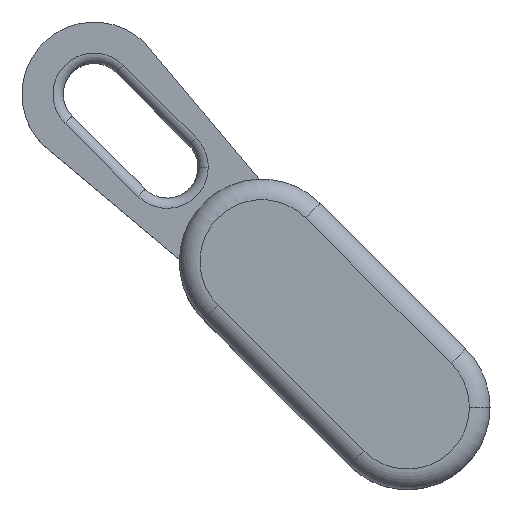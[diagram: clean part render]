
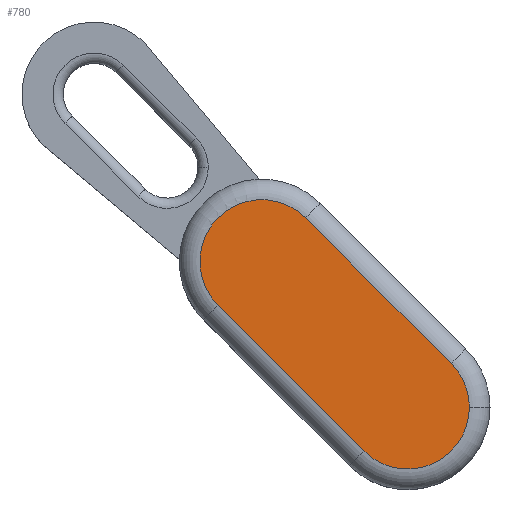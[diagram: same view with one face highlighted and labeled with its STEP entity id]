
A CAD part, top view. The second image highlights one B-rep face of the part: STEP entity #780.
In plain terms, the highlighted planar face has unit normal (0, 0, 1).
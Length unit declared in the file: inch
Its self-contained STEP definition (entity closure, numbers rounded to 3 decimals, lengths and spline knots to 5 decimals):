
#4 = LINE ( 'NONE', #645, #909 ) ;
#46 = FACE_OUTER_BOUND ( 'NONE', #1420, .T. ) ;
#127 = DIRECTION ( 'NONE',  ( 0.707, -0.707, 0. ) ) ;
#155 = VERTEX_POINT ( 'NONE', #1079 ) ;
#251 = DIRECTION ( 'NONE',  ( 0., 0., 1. ) ) ;
#254 = CIRCLE ( 'NONE', #668, 0.11811 ) ;
#264 = EDGE_CURVE ( 'NONE', #755, #1204, #975, .T. ) ;
#313 = DIRECTION ( 'NONE',  ( 0., 0., 1. ) ) ;
#320 = CARTESIAN_POINT ( 'NONE',  ( 0.55657, -0.50477, 0.61024 ) ) ;
#396 = CARTESIAN_POINT ( 'NONE',  ( 0.16007, -0.22638, 0.61024 ) ) ;
#404 = DIRECTION ( 'NONE',  ( 0., 0., 1. ) ) ;
#526 = DIRECTION ( 'NONE',  ( 1., 0., 0. ) ) ;
#633 = LINE ( 'NONE', #1086, #1436 ) ;
#645 = CARTESIAN_POINT ( 'NONE',  ( 0.05036, 0.05036, 0.61024 ) ) ;
#668 = AXIS2_PLACEMENT_3D ( 'NONE', #1092, #404, #1200 ) ;
#702 = AXIS2_PLACEMENT_3D ( 'NONE', #396, #1196, #526 ) ;
#755 = VERTEX_POINT ( 'NONE', #1172 ) ;
#763 = DIRECTION ( 'NONE',  ( -0.707, 0.707, 0. ) ) ;
#780 = ADVANCED_FACE ( 'NONE', ( #46 ), #971, .T. ) ;
#805 = EDGE_CURVE ( 'NONE', #1356, #155, #4, .T. ) ;
#812 = EDGE_CURVE ( 'NONE', #155, #1235, #1184, .T. ) ;
#817 = EDGE_CURVE ( 'NONE', #1235, #755, #633, .T. ) ;
#835 = EDGE_CURVE ( 'NONE', #1204, #1356, #254, .T. ) ;
#867 = CARTESIAN_POINT ( 'NONE',  ( 0., 0., 0.61024 ) ) ;
#909 = VECTOR ( 'NONE', #763, 39.37008 ) ;
#920 = ORIENTED_EDGE ( 'NONE', *, *, #264, .T. ) ;
#952 = ORIENTED_EDGE ( 'NONE', *, *, #805, .T. ) ;
#964 = AXIS2_PLACEMENT_3D ( 'NONE', #867, #251, #1077 ) ;
#971 = PLANE ( 'NONE',  #964 ) ;
#975 = CIRCLE ( 'NONE', #1213, 0.11811 ) ;
#1021 = CARTESIAN_POINT ( 'NONE',  ( 0.43846, -0.50477, 0.61024 ) ) ;
#1033 = CARTESIAN_POINT ( 'NONE',  ( 0.07656, -0.30989, 0.61024 ) ) ;
#1076 = ORIENTED_EDGE ( 'NONE', *, *, #817, .T. ) ;
#1077 = DIRECTION ( 'NONE',  ( 1., 0., 0. ) ) ;
#1079 = CARTESIAN_POINT ( 'NONE',  ( 0.24359, -0.14286, 0.61024 ) ) ;
#1086 = CARTESIAN_POINT ( 'NONE',  ( 0.35495, -0.58828, 0.61024 ) ) ;
#1092 = CARTESIAN_POINT ( 'NONE',  ( 0.43846, -0.50477, 0.61024 ) ) ;
#1128 = DIRECTION ( 'NONE',  ( 1., 0., 0. ) ) ;
#1162 = ORIENTED_EDGE ( 'NONE', *, *, #835, .T. ) ;
#1172 = CARTESIAN_POINT ( 'NONE',  ( 0.35495, -0.58828, 0.61024 ) ) ;
#1179 = ORIENTED_EDGE ( 'NONE', *, *, #812, .T. ) ;
#1184 = CIRCLE ( 'NONE', #702, 0.11811 ) ;
#1196 = DIRECTION ( 'NONE',  ( 0., 0., 1. ) ) ;
#1200 = DIRECTION ( 'NONE',  ( 1., 0., 0. ) ) ;
#1204 = VERTEX_POINT ( 'NONE', #320 ) ;
#1213 = AXIS2_PLACEMENT_3D ( 'NONE', #1021, #313, #1128 ) ;
#1235 = VERTEX_POINT ( 'NONE', #1033 ) ;
#1355 = CARTESIAN_POINT ( 'NONE',  ( 0.52198, -0.42125, 0.61024 ) ) ;
#1356 = VERTEX_POINT ( 'NONE', #1355 ) ;
#1420 = EDGE_LOOP ( 'NONE', ( #952, #1179, #1076, #920, #1162 ) ) ;
#1436 = VECTOR ( 'NONE', #127, 39.37008 ) ;
